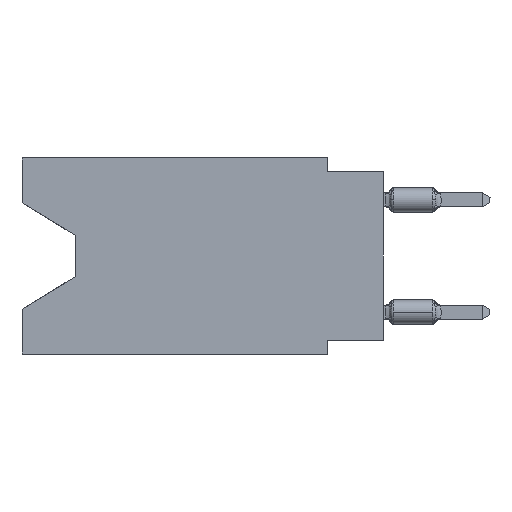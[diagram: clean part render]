
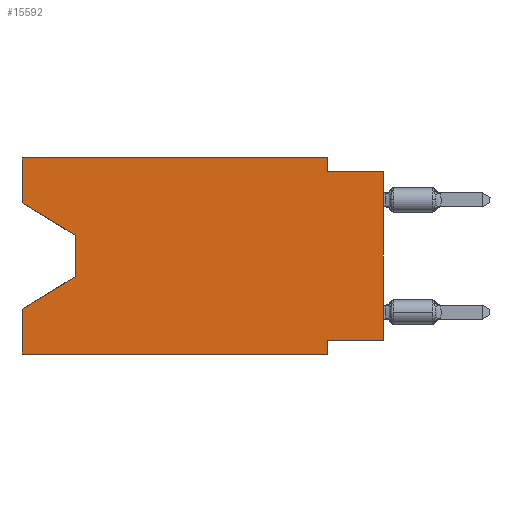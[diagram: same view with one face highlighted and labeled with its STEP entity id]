
A CAD part, left-side view. The second image highlights one B-rep face of the part: STEP entity #15592.
In plain terms, the highlighted planar face has unit normal (-1, 0, 0).
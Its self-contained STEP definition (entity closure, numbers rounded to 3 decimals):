
#397 = CARTESIAN_POINT ( 'NONE',  ( 0., 2.54, 0. ) ) ;
#709 = VECTOR ( 'NONE', #21553, 1000. ) ;
#1015 = VERTEX_POINT ( 'NONE', #397 ) ;
#1403 = CARTESIAN_POINT ( 'NONE',  ( 0., 13.97, -5.385 ) ) ;
#2541 = LINE ( 'NONE', #28246, #33993 ) ;
#2941 = VECTOR ( 'NONE', #33284, 1000. ) ;
#3366 = VERTEX_POINT ( 'NONE', #10330 ) ;
#3456 = VERTEX_POINT ( 'NONE', #17859 ) ;
#4510 = VERTEX_POINT ( 'NONE', #4517 ) ;
#4517 = CARTESIAN_POINT ( 'NONE',  ( 0., 16.383, -2.038 ) ) ;
#4891 = VERTEX_POINT ( 'NONE', #38511 ) ;
#4959 = VECTOR ( 'NONE', #7987, 1000. ) ;
#5006 = ORIENTED_EDGE ( 'NONE', *, *, #31266, .F. ) ;
#5039 = VECTOR ( 'NONE', #5887, 1000. ) ;
#5366 = VERTEX_POINT ( 'NONE', #17137 ) ;
#5562 = ORIENTED_EDGE ( 'NONE', *, *, #21661, .T. ) ;
#5887 = DIRECTION ( 'NONE',  ( 0., 0., -1. ) ) ;
#5907 = CARTESIAN_POINT ( 'NONE',  ( 0., 16.383, 0. ) ) ;
#6098 = VECTOR ( 'NONE', #14808, 1000. ) ;
#6344 = DIRECTION ( 'NONE',  ( 0., 0., -1. ) ) ;
#6765 = CARTESIAN_POINT ( 'NONE',  ( 0., 13.97, -3.505 ) ) ;
#7055 = VERTEX_POINT ( 'NONE', #1403 ) ;
#7797 = VERTEX_POINT ( 'NONE', #6765 ) ;
#7803 = LINE ( 'NONE', #20563, #2941 ) ;
#7987 = DIRECTION ( 'NONE',  ( 0., -1., 0. ) ) ;
#8634 = CARTESIAN_POINT ( 'NONE',  ( 0., 13.97, -5.385 ) ) ;
#8849 = EDGE_CURVE ( 'NONE', #11487, #27427, #11704, .T. ) ;
#9434 = DIRECTION ( 'NONE',  ( 0., 0., 1. ) ) ;
#9442 = EDGE_CURVE ( 'NONE', #5366, #4891, #26010, .T. ) ;
#9471 = CARTESIAN_POINT ( 'NONE',  ( 0., 13.97, -3.505 ) ) ;
#9568 = VECTOR ( 'NONE', #35963, 1000. ) ;
#9606 = ORIENTED_EDGE ( 'NONE', *, *, #14736, .F. ) ;
#9900 = CARTESIAN_POINT ( 'NONE',  ( 0., 16.383, -8.89 ) ) ;
#10270 = ORIENTED_EDGE ( 'NONE', *, *, #38390, .F. ) ;
#10330 = CARTESIAN_POINT ( 'NONE',  ( 0., 16.383, -6.852 ) ) ;
#11487 = VERTEX_POINT ( 'NONE', #16718 ) ;
#11704 = LINE ( 'NONE', #24470, #709 ) ;
#14268 = CARTESIAN_POINT ( 'NONE',  ( 0., 0., -0.635 ) ) ;
#14354 = ORIENTED_EDGE ( 'NONE', *, *, #17598, .F. ) ;
#14602 = CARTESIAN_POINT ( 'NONE',  ( 0., 2.54, 0. ) ) ;
#14664 = FACE_OUTER_BOUND ( 'NONE', #14923, .T. ) ;
#14736 = EDGE_CURVE ( 'NONE', #1015, #3456, #17743, .T. ) ;
#14808 = DIRECTION ( 'NONE',  ( 0., 0., -1. ) ) ;
#14923 = EDGE_LOOP ( 'NONE', ( #5562, #18594, #19145, #10270, #28347, #23984, #5006, #40430, #24388, #9606, #14354, #31671 ) ) ;
#15114 = VECTOR ( 'NONE', #6344, 1000. ) ;
#15592 = ADVANCED_FACE ( 'NONE', ( #14664 ), #24893, .F. ) ;
#15698 = CARTESIAN_POINT ( 'NONE',  ( 0., 2.54, -8.89 ) ) ;
#16718 = CARTESIAN_POINT ( 'NONE',  ( 0., 0., -8.255 ) ) ;
#16993 = LINE ( 'NONE', #14268, #4959 ) ;
#17137 = CARTESIAN_POINT ( 'NONE',  ( 0., 16.383, -8.89 ) ) ;
#17598 = EDGE_CURVE ( 'NONE', #38515, #1015, #25299, .T. ) ;
#17743 = LINE ( 'NONE', #14602, #6098 ) ;
#17859 = CARTESIAN_POINT ( 'NONE',  ( 0., 2.54, -0.635 ) ) ;
#18218 = DIRECTION ( 'NONE',  ( 1., 0., 0. ) ) ;
#18439 = DIRECTION ( 'NONE',  ( 0., 0., 1. ) ) ;
#18594 = ORIENTED_EDGE ( 'NONE', *, *, #28638, .T. ) ;
#18703 = EDGE_CURVE ( 'NONE', #7055, #3366, #37263, .T. ) ;
#19073 = LINE ( 'NONE', #5907, #27586 ) ;
#19145 = ORIENTED_EDGE ( 'NONE', *, *, #18703, .T. ) ;
#19367 = VERTEX_POINT ( 'NONE', #36910 ) ;
#19943 = DIRECTION ( 'NONE',  ( 0., -1., 0. ) ) ;
#20563 = CARTESIAN_POINT ( 'NONE',  ( 0., 0., -8.255 ) ) ;
#20795 = VECTOR ( 'NONE', #28079, 1000. ) ;
#21553 = DIRECTION ( 'NONE',  ( 0., 0., 1. ) ) ;
#21661 = EDGE_CURVE ( 'NONE', #4510, #7797, #29071, .T. ) ;
#22173 = CARTESIAN_POINT ( 'NONE',  ( 0., 16.383, 0. ) ) ;
#22607 = LINE ( 'NONE', #15698, #5039 ) ;
#22643 = EDGE_CURVE ( 'NONE', #4510, #38515, #19073, .T. ) ;
#23984 = ORIENTED_EDGE ( 'NONE', *, *, #34288, .F. ) ;
#24053 = EDGE_CURVE ( 'NONE', #3456, #27427, #16993, .T. ) ;
#24388 = ORIENTED_EDGE ( 'NONE', *, *, #24053, .F. ) ;
#24470 = CARTESIAN_POINT ( 'NONE',  ( 0., 0., 0. ) ) ;
#24893 = PLANE ( 'NONE',  #28622 ) ;
#25299 = LINE ( 'NONE', #22173, #39073 ) ;
#25453 = VECTOR ( 'NONE', #19943, 1000. ) ;
#26010 = LINE ( 'NONE', #9900, #25453 ) ;
#27410 = DIRECTION ( 'NONE',  ( 0., 0., -1. ) ) ;
#27427 = VERTEX_POINT ( 'NONE', #31230 ) ;
#27586 = VECTOR ( 'NONE', #9434, 1000. ) ;
#28079 = DIRECTION ( 'NONE',  ( 0., 0.855, -0.519 ) ) ;
#28246 = CARTESIAN_POINT ( 'NONE',  ( 0., 16.383, 0. ) ) ;
#28347 = ORIENTED_EDGE ( 'NONE', *, *, #9442, .T. ) ;
#28622 = AXIS2_PLACEMENT_3D ( 'NONE', #34075, #18218, #27410 ) ;
#28638 = EDGE_CURVE ( 'NONE', #7797, #7055, #38118, .T. ) ;
#29071 = LINE ( 'NONE', #32813, #9568 ) ;
#31230 = CARTESIAN_POINT ( 'NONE',  ( 0., 0., -0.635 ) ) ;
#31266 = EDGE_CURVE ( 'NONE', #11487, #19367, #7803, .T. ) ;
#31671 = ORIENTED_EDGE ( 'NONE', *, *, #22643, .F. ) ;
#32813 = CARTESIAN_POINT ( 'NONE',  ( 0., 16.383, -2.038 ) ) ;
#33284 = DIRECTION ( 'NONE',  ( 0., 1., 0. ) ) ;
#33993 = VECTOR ( 'NONE', #18439, 1000. ) ;
#34075 = CARTESIAN_POINT ( 'NONE',  ( 0., 16.383, 0. ) ) ;
#34288 = EDGE_CURVE ( 'NONE', #19367, #4891, #22607, .T. ) ;
#34882 = DIRECTION ( 'NONE',  ( 0., -1., 0. ) ) ;
#35537 = CARTESIAN_POINT ( 'NONE',  ( 0., 16.383, 0. ) ) ;
#35963 = DIRECTION ( 'NONE',  ( 0., -0.855, -0.519 ) ) ;
#36910 = CARTESIAN_POINT ( 'NONE',  ( 0., 2.54, -8.255 ) ) ;
#37263 = LINE ( 'NONE', #8634, #20795 ) ;
#38118 = LINE ( 'NONE', #9471, #15114 ) ;
#38390 = EDGE_CURVE ( 'NONE', #5366, #3366, #2541, .T. ) ;
#38511 = CARTESIAN_POINT ( 'NONE',  ( 0., 2.54, -8.89 ) ) ;
#38515 = VERTEX_POINT ( 'NONE', #35537 ) ;
#39073 = VECTOR ( 'NONE', #34882, 1000. ) ;
#40430 = ORIENTED_EDGE ( 'NONE', *, *, #8849, .T. ) ;
